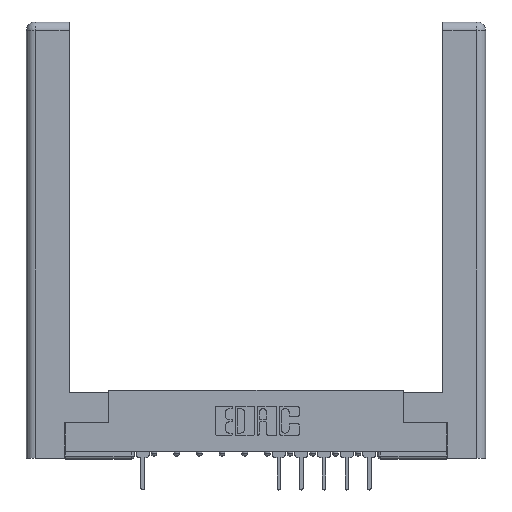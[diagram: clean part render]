
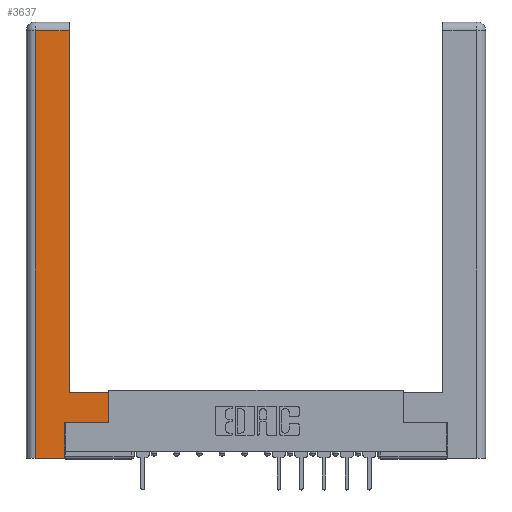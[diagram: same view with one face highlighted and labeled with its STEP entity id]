
A CAD part, top view. The second image highlights one B-rep face of the part: STEP entity #3637.
In plain terms, the highlighted planar face has unit normal (0, 0, 1).
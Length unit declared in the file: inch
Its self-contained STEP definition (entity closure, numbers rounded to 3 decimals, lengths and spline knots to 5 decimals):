
#154 = CARTESIAN_POINT ( 'NONE',  ( 0.295, 0.45, 0. ) ) ;
#529 = ORIENTED_EDGE ( 'NONE', *, *, #8963, .T. ) ;
#533 = CARTESIAN_POINT ( 'NONE',  ( 0.0615, 2.94, 0. ) ) ;
#665 = EDGE_CURVE ( 'NONE', #2633, #8668, #8450, .T. ) ;
#710 = EDGE_CURVE ( 'NONE', #1034, #12554, #1143, .T. ) ;
#1034 = VERTEX_POINT ( 'NONE', #6884 ) ;
#1051 = VECTOR ( 'NONE', #7892, 39.37008 ) ;
#1143 = LINE ( 'NONE', #154, #14068 ) ;
#1323 = CARTESIAN_POINT ( 'NONE',  ( 0.565, 0.45, 0. ) ) ;
#1588 = CARTESIAN_POINT ( 'NONE',  ( 0.295, 0.45, 0. ) ) ;
#1791 = CARTESIAN_POINT ( 'NONE',  ( 0.0615, 2.94, 0. ) ) ;
#1892 = ORIENTED_EDGE ( 'NONE', *, *, #710, .T. ) ;
#2633 = VERTEX_POINT ( 'NONE', #13730 ) ;
#2720 = EDGE_CURVE ( 'NONE', #7882, #3622, #7808, .T. ) ;
#2798 = VECTOR ( 'NONE', #12469, 39.37008 ) ;
#3054 = CARTESIAN_POINT ( 'NONE',  ( 0.295, 2.94, 0. ) ) ;
#3113 = VERTEX_POINT ( 'NONE', #9918 ) ;
#3364 = EDGE_CURVE ( 'NONE', #8514, #3113, #7594, .T. ) ;
#3420 = ORIENTED_EDGE ( 'NONE', *, *, #2720, .T. ) ;
#3622 = VERTEX_POINT ( 'NONE', #533 ) ;
#3637 = ADVANCED_FACE ( 'NONE', ( #10248 ), #5451, .F. ) ;
#3974 = EDGE_LOOP ( 'NONE', ( #3995, #3420, #15361, #14896, #529, #6330, #10726, #1892 ) ) ;
#3995 = ORIENTED_EDGE ( 'NONE', *, *, #12958, .T. ) ;
#4509 = VECTOR ( 'NONE', #9139, 39.37008 ) ;
#5451 = PLANE ( 'NONE',  #13305 ) ;
#6248 = DIRECTION ( 'NONE',  ( 0., 1., 0. ) ) ;
#6330 = ORIENTED_EDGE ( 'NONE', *, *, #665, .T. ) ;
#6662 = CARTESIAN_POINT ( 'NONE',  ( 0.265, 0., 0. ) ) ;
#6728 = DIRECTION ( 'NONE',  ( 0., 0., -1. ) ) ;
#6884 = CARTESIAN_POINT ( 'NONE',  ( 0.565, 0.45, 0. ) ) ;
#6895 = LINE ( 'NONE', #14392, #12933 ) ;
#7396 = VECTOR ( 'NONE', #7491, 39.37008 ) ;
#7491 = DIRECTION ( 'NONE',  ( 0., 1., 0. ) ) ;
#7594 = LINE ( 'NONE', #6662, #1051 ) ;
#7785 = VECTOR ( 'NONE', #6248, 39.37008 ) ;
#7808 = LINE ( 'NONE', #1791, #4509 ) ;
#7882 = VERTEX_POINT ( 'NONE', #3054 ) ;
#7892 = DIRECTION ( 'NONE',  ( 1., 0., 0. ) ) ;
#8381 = EDGE_CURVE ( 'NONE', #3622, #8514, #12524, .T. ) ;
#8442 = DIRECTION ( 'NONE',  ( 0., 1., 0. ) ) ;
#8450 = LINE ( 'NONE', #12243, #11295 ) ;
#8514 = VERTEX_POINT ( 'NONE', #12719 ) ;
#8668 = VERTEX_POINT ( 'NONE', #10576 ) ;
#8725 = DIRECTION ( 'NONE',  ( -1., 0., 0. ) ) ;
#8934 = EDGE_CURVE ( 'NONE', #8668, #1034, #14157, .T. ) ;
#8963 = EDGE_CURVE ( 'NONE', #3113, #2633, #13795, .T. ) ;
#9139 = DIRECTION ( 'NONE',  ( -1., 0., 0. ) ) ;
#9918 = CARTESIAN_POINT ( 'NONE',  ( 0.265, 0., 0. ) ) ;
#10248 = FACE_OUTER_BOUND ( 'NONE', #3974, .T. ) ;
#10576 = CARTESIAN_POINT ( 'NONE',  ( 0.565, 0.245, 0. ) ) ;
#10726 = ORIENTED_EDGE ( 'NONE', *, *, #8934, .T. ) ;
#11279 = CARTESIAN_POINT ( 'NONE',  ( 0.0615, 0., 0. ) ) ;
#11295 = VECTOR ( 'NONE', #13422, 39.37008 ) ;
#12243 = CARTESIAN_POINT ( 'NONE',  ( 0.565, 0.245, 0. ) ) ;
#12469 = DIRECTION ( 'NONE',  ( 0., -1., 0. ) ) ;
#12524 = LINE ( 'NONE', #11279, #2798 ) ;
#12554 = VERTEX_POINT ( 'NONE', #1588 ) ;
#12719 = CARTESIAN_POINT ( 'NONE',  ( 0.0615, 0., 0. ) ) ;
#12933 = VECTOR ( 'NONE', #8442, 39.37008 ) ;
#12958 = EDGE_CURVE ( 'NONE', #12554, #7882, #6895, .T. ) ;
#13305 = AXIS2_PLACEMENT_3D ( 'NONE', #13940, #6728, #15099 ) ;
#13422 = DIRECTION ( 'NONE',  ( 1., 0., 0. ) ) ;
#13530 = CARTESIAN_POINT ( 'NONE',  ( 0.265, 0.245, 0. ) ) ;
#13730 = CARTESIAN_POINT ( 'NONE',  ( 0.265, 0.245, 0. ) ) ;
#13795 = LINE ( 'NONE', #13530, #7396 ) ;
#13940 = CARTESIAN_POINT ( 'NONE',  ( 0., 0., 0. ) ) ;
#14068 = VECTOR ( 'NONE', #8725, 39.37008 ) ;
#14157 = LINE ( 'NONE', #1323, #7785 ) ;
#14392 = CARTESIAN_POINT ( 'NONE',  ( 0.295, 3., 0. ) ) ;
#14896 = ORIENTED_EDGE ( 'NONE', *, *, #3364, .T. ) ;
#15099 = DIRECTION ( 'NONE',  ( -1., 0., 0. ) ) ;
#15361 = ORIENTED_EDGE ( 'NONE', *, *, #8381, .T. ) ;
